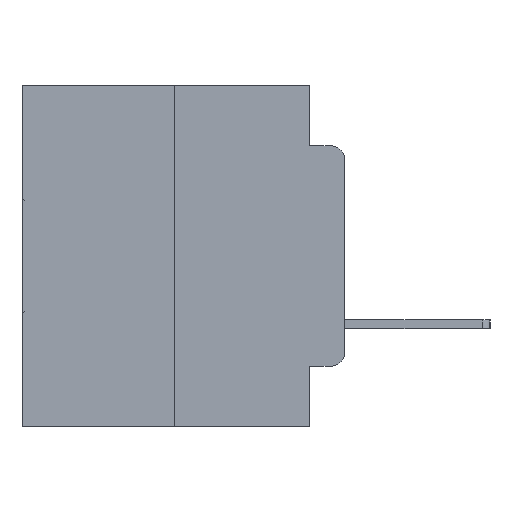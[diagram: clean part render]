
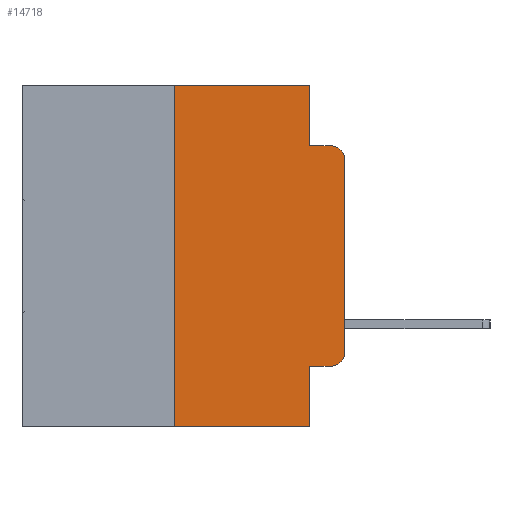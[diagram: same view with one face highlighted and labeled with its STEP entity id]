
A CAD part, left-side view. The second image highlights one B-rep face of the part: STEP entity #14718.
In plain terms, the highlighted planar face has unit normal (-1, 0, 0).
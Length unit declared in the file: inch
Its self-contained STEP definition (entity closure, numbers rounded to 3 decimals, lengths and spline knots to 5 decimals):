
#65 = AXIS2_PLACEMENT_3D ( 'NONE', #19816, #2161, #5659 ) ;
#71 = ORIENTED_EDGE ( 'NONE', *, *, #681, .F. ) ;
#221 = VECTOR ( 'NONE', #2601, 39.37008 ) ;
#411 = EDGE_CURVE ( 'NONE', #28806, #16324, #14498, .T. ) ;
#463 = EDGE_CURVE ( 'NONE', #12409, #28806, #24035, .T. ) ;
#503 = EDGE_CURVE ( 'NONE', #12409, #25242, #11040, .T. ) ;
#547 = EDGE_CURVE ( 'NONE', #1404, #3854, #2862, .T. ) ;
#552 = EDGE_CURVE ( 'NONE', #15196, #3433, #19279, .T. ) ;
#681 = EDGE_CURVE ( 'NONE', #1343, #15196, #1759, .T. ) ;
#690 = EDGE_CURVE ( 'NONE', #16324, #3881, #18238, .T. ) ;
#724 = EDGE_CURVE ( 'NONE', #3881, #3433, #5747, .T. ) ;
#1056 = FACE_OUTER_BOUND ( 'NONE', #25548, .T. ) ;
#1128 = CARTESIAN_POINT ( 'NONE',  ( 0., 0.02, -0.4115 ) ) ;
#1343 = VERTEX_POINT ( 'NONE', #18082 ) ;
#1404 = VERTEX_POINT ( 'NONE', #18454 ) ;
#1532 = CARTESIAN_POINT ( 'NONE',  ( 0., 0., -0.3915 ) ) ;
#1759 = LINE ( 'NONE', #12788, #24681 ) ;
#1815 = DIRECTION ( 'NONE',  ( 0., -1., 0. ) ) ;
#2161 = DIRECTION ( 'NONE',  ( -1., 0., 0. ) ) ;
#2601 = DIRECTION ( 'NONE',  ( 0., 0., 1. ) ) ;
#2828 = PLANE ( 'NONE',  #17110 ) ;
#2862 = LINE ( 'NONE', #26051, #8249 ) ;
#3409 = VECTOR ( 'NONE', #1815, 39.37008 ) ;
#3433 = VERTEX_POINT ( 'NONE', #7311 ) ;
#3754 = ORIENTED_EDGE ( 'NONE', *, *, #411, .T. ) ;
#3854 = VERTEX_POINT ( 'NONE', #13802 ) ;
#3881 = VERTEX_POINT ( 'NONE', #9589 ) ;
#5659 = DIRECTION ( 'NONE',  ( 0., 0., -1. ) ) ;
#5747 = CIRCLE ( 'NONE', #65, 0.02 ) ;
#6731 = CARTESIAN_POINT ( 'NONE',  ( 0., 0.051, -0.0885 ) ) ;
#7311 = CARTESIAN_POINT ( 'NONE',  ( 0., 0.02, -0.0885 ) ) ;
#8249 = VECTOR ( 'NONE', #12111, 39.37008 ) ;
#8394 = LINE ( 'NONE', #16150, #18725 ) ;
#8986 = CARTESIAN_POINT ( 'NONE',  ( 0., 0.051, -0.0885 ) ) ;
#9589 = CARTESIAN_POINT ( 'NONE',  ( 0., 0., -0.1085 ) ) ;
#9744 = DIRECTION ( 'NONE',  ( 0., 0., -1. ) ) ;
#11040 = LINE ( 'NONE', #26820, #21991 ) ;
#11719 = VECTOR ( 'NONE', #20491, 39.37008 ) ;
#11978 = EDGE_CURVE ( 'NONE', #3854, #1343, #15348, .T. ) ;
#12111 = DIRECTION ( 'NONE',  ( 0., 0., 1. ) ) ;
#12409 = VERTEX_POINT ( 'NONE', #25270 ) ;
#12788 = CARTESIAN_POINT ( 'NONE',  ( 0., 0.051, 0. ) ) ;
#13282 = ORIENTED_EDGE ( 'NONE', *, *, #11978, .F. ) ;
#13450 = VECTOR ( 'NONE', #26688, 39.37008 ) ;
#13754 = ORIENTED_EDGE ( 'NONE', *, *, #690, .T. ) ;
#13802 = CARTESIAN_POINT ( 'NONE',  ( 0., 0.25, 0. ) ) ;
#14498 = CIRCLE ( 'NONE', #28553, 0.02 ) ;
#14718 = ADVANCED_FACE ( 'NONE', ( #1056 ), #2828, .F. ) ;
#14991 = ORIENTED_EDGE ( 'NONE', *, *, #503, .F. ) ;
#15196 = VERTEX_POINT ( 'NONE', #6731 ) ;
#15348 = LINE ( 'NONE', #19694, #3409 ) ;
#16150 = CARTESIAN_POINT ( 'NONE',  ( 0., 0.473, -0.5 ) ) ;
#16324 = VERTEX_POINT ( 'NONE', #1532 ) ;
#17110 = AXIS2_PLACEMENT_3D ( 'NONE', #20620, #22823, #9744 ) ;
#18082 = CARTESIAN_POINT ( 'NONE',  ( 0., 0.051, 0. ) ) ;
#18238 = LINE ( 'NONE', #23154, #221 ) ;
#18358 = DIRECTION ( 'NONE',  ( 0., -1., 0. ) ) ;
#18454 = CARTESIAN_POINT ( 'NONE',  ( 0., 0.25, -0.5 ) ) ;
#18725 = VECTOR ( 'NONE', #18358, 39.37008 ) ;
#18779 = ORIENTED_EDGE ( 'NONE', *, *, #552, .F. ) ;
#19279 = LINE ( 'NONE', #8986, #13450 ) ;
#19694 = CARTESIAN_POINT ( 'NONE',  ( 0., 0.473, 0. ) ) ;
#19816 = CARTESIAN_POINT ( 'NONE',  ( 0., 0.02, -0.1085 ) ) ;
#20491 = DIRECTION ( 'NONE',  ( 0., -1., 0. ) ) ;
#20620 = CARTESIAN_POINT ( 'NONE',  ( 0., 0.473, 0. ) ) ;
#20777 = ORIENTED_EDGE ( 'NONE', *, *, #26702, .T. ) ;
#21991 = VECTOR ( 'NONE', #24736, 39.37008 ) ;
#21996 = CARTESIAN_POINT ( 'NONE',  ( 0., 0.02, -0.3915 ) ) ;
#22123 = ORIENTED_EDGE ( 'NONE', *, *, #463, .T. ) ;
#22195 = ORIENTED_EDGE ( 'NONE', *, *, #724, .T. ) ;
#22224 = DIRECTION ( 'NONE',  ( 0., 0., -1. ) ) ;
#22370 = DIRECTION ( 'NONE',  ( -1., 0., 0. ) ) ;
#22823 = DIRECTION ( 'NONE',  ( 1., 0., 0. ) ) ;
#23154 = CARTESIAN_POINT ( 'NONE',  ( 0., 0., 0. ) ) ;
#24035 = LINE ( 'NONE', #26140, #11719 ) ;
#24681 = VECTOR ( 'NONE', #27161, 39.37008 ) ;
#24736 = DIRECTION ( 'NONE',  ( 0., 0., -1. ) ) ;
#25242 = VERTEX_POINT ( 'NONE', #27574 ) ;
#25270 = CARTESIAN_POINT ( 'NONE',  ( 0., 0.051, -0.4115 ) ) ;
#25548 = EDGE_LOOP ( 'NONE', ( #13754, #22195, #18779, #71, #13282, #27233, #20777, #14991, #22123, #3754 ) ) ;
#26051 = CARTESIAN_POINT ( 'NONE',  ( 0., 0.25, 0. ) ) ;
#26140 = CARTESIAN_POINT ( 'NONE',  ( 0., 0.051, -0.4115 ) ) ;
#26688 = DIRECTION ( 'NONE',  ( 0., -1., 0. ) ) ;
#26702 = EDGE_CURVE ( 'NONE', #1404, #25242, #8394, .T. ) ;
#26820 = CARTESIAN_POINT ( 'NONE',  ( 0., 0.051, 0. ) ) ;
#27161 = DIRECTION ( 'NONE',  ( 0., 0., -1. ) ) ;
#27233 = ORIENTED_EDGE ( 'NONE', *, *, #547, .F. ) ;
#27574 = CARTESIAN_POINT ( 'NONE',  ( 0., 0.051, -0.5 ) ) ;
#28553 = AXIS2_PLACEMENT_3D ( 'NONE', #21996, #22370, #22224 ) ;
#28806 = VERTEX_POINT ( 'NONE', #1128 ) ;
